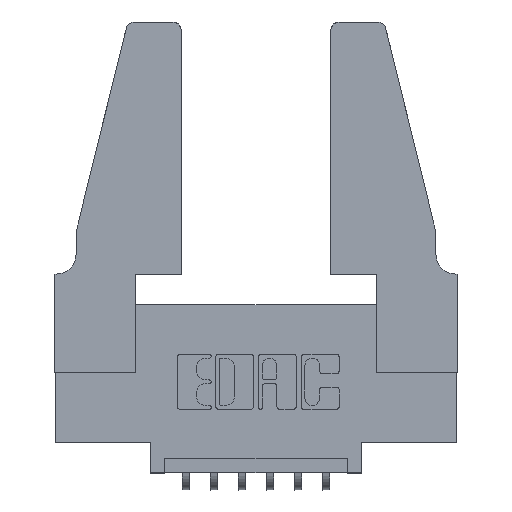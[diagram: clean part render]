
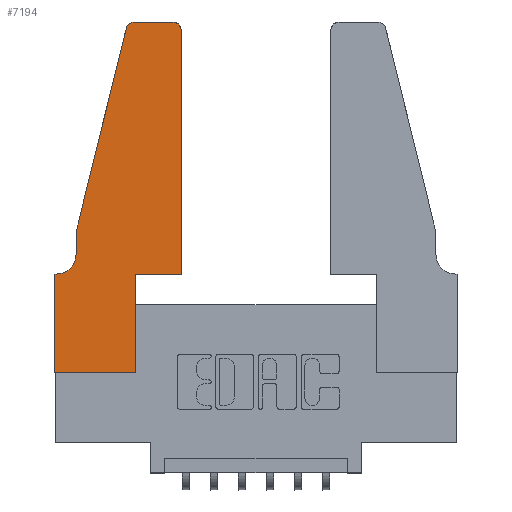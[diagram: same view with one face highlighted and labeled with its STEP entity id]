
A CAD part, top view. The second image highlights one B-rep face of the part: STEP entity #7194.
In plain terms, the highlighted planar face has unit normal (0, 0, 1).
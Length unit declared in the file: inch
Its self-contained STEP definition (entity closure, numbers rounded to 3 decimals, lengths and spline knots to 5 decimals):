
#24 = VECTOR ( 'NONE', #1150, 39.37008 ) ;
#95 = VECTOR ( 'NONE', #7363, 39.37008 ) ;
#109 = VERTEX_POINT ( 'NONE', #2676 ) ;
#180 = CARTESIAN_POINT ( 'NONE',  ( 0.25487, 1.22718, 0.37 ) ) ;
#344 = VERTEX_POINT ( 'NONE', #8142 ) ;
#568 = LINE ( 'NONE', #11033, #24 ) ;
#684 = ORIENTED_EDGE ( 'NONE', *, *, #7109, .T. ) ;
#861 = EDGE_CURVE ( 'NONE', #4608, #11034, #10524, .T. ) ;
#990 = ORIENTED_EDGE ( 'NONE', *, *, #3376, .T. ) ;
#1132 = CARTESIAN_POINT ( 'NONE',  ( 0.0755, 0.5, 0.37 ) ) ;
#1150 = DIRECTION ( 'NONE',  ( -1., 0., 0. ) ) ;
#1303 = VECTOR ( 'NONE', #10453, 39.37008 ) ;
#1322 = VERTEX_POINT ( 'NONE', #3281 ) ;
#1343 = EDGE_CURVE ( 'NONE', #11439, #109, #3256, .T. ) ;
#1404 = CARTESIAN_POINT ( 'NONE',  ( 0.4205, 1.22, 0.37 ) ) ;
#1471 = ORIENTED_EDGE ( 'NONE', *, *, #6889, .T. ) ;
#1481 = DIRECTION ( 'NONE',  ( 1., 0., 0. ) ) ;
#1549 = DIRECTION ( 'NONE',  ( 1., 0., 0. ) ) ;
#1563 = LINE ( 'NONE', #1868, #9093 ) ;
#1603 = VERTEX_POINT ( 'NONE', #1836 ) ;
#1688 = ORIENTED_EDGE ( 'NONE', *, *, #11092, .T. ) ;
#1743 = EDGE_CURVE ( 'NONE', #1603, #4608, #568, .T. ) ;
#1781 = CARTESIAN_POINT ( 'NONE',  ( 0.0755, 0.35, 0.37 ) ) ;
#1814 = EDGE_CURVE ( 'NONE', #1917, #1603, #8633, .T. ) ;
#1836 = CARTESIAN_POINT ( 'NONE',  ( 0.4205, 1.25, 0.37 ) ) ;
#1868 = CARTESIAN_POINT ( 'NONE',  ( 0., 0., 0.37 ) ) ;
#1917 = VERTEX_POINT ( 'NONE', #6999 ) ;
#2263 = CARTESIAN_POINT ( 'NONE',  ( 0.4505, 0.35, 0.37 ) ) ;
#2401 = PLANE ( 'NONE',  #6194 ) ;
#2641 = EDGE_CURVE ( 'NONE', #7543, #344, #9566, .T. ) ;
#2676 = CARTESIAN_POINT ( 'NONE',  ( 0.2865, 0., 0.37 ) ) ;
#2897 = CARTESIAN_POINT ( 'NONE',  ( 0.0755, 0.5, 0.37 ) ) ;
#2958 = VERTEX_POINT ( 'NONE', #1132 ) ;
#3074 = VERTEX_POINT ( 'NONE', #2263 ) ;
#3115 = EDGE_CURVE ( 'NONE', #109, #1322, #11562, .T. ) ;
#3256 = LINE ( 'NONE', #10674, #9085 ) ;
#3281 = CARTESIAN_POINT ( 'NONE',  ( 0.2865, 0.35, 0.37 ) ) ;
#3353 = ORIENTED_EDGE ( 'NONE', *, *, #1743, .T. ) ;
#3376 = EDGE_CURVE ( 'NONE', #2958, #7543, #3465, .T. ) ;
#3465 = LINE ( 'NONE', #2897, #95 ) ;
#3776 = EDGE_LOOP ( 'NONE', ( #3353, #9529, #4722, #990, #9411, #1471, #10688, #6001, #7278, #1688, #684, #6010 ) ) ;
#4322 = AXIS2_PLACEMENT_3D ( 'NONE', #6263, #8201, #4456 ) ;
#4456 = DIRECTION ( 'NONE',  ( -1., 0., 0. ) ) ;
#4553 = VECTOR ( 'NONE', #5973, 39.37008 ) ;
#4608 = VERTEX_POINT ( 'NONE', #6114 ) ;
#4722 = ORIENTED_EDGE ( 'NONE', *, *, #5893, .T. ) ;
#5148 = CARTESIAN_POINT ( 'NONE',  ( 0.0755, 0.5, 0.37 ) ) ;
#5365 = CARTESIAN_POINT ( 'NONE',  ( 0., 0., 0.37 ) ) ;
#5893 = EDGE_CURVE ( 'NONE', #11034, #2958, #7046, .T. ) ;
#5973 = DIRECTION ( 'NONE',  ( -0.239, -0.971, 0. ) ) ;
#6001 = ORIENTED_EDGE ( 'NONE', *, *, #1343, .T. ) ;
#6010 = ORIENTED_EDGE ( 'NONE', *, *, #1814, .T. ) ;
#6114 = CARTESIAN_POINT ( 'NONE',  ( 0.284, 1.25, 0.37 ) ) ;
#6194 = AXIS2_PLACEMENT_3D ( 'NONE', #11476, #9699, #8766 ) ;
#6263 = CARTESIAN_POINT ( 'NONE',  ( 0.0055, 0.42, 0.37 ) ) ;
#6622 = VECTOR ( 'NONE', #9454, 39.37008 ) ;
#6735 = CARTESIAN_POINT ( 'NONE',  ( 0.284, 1.22, 0.37 ) ) ;
#6889 = EDGE_CURVE ( 'NONE', #344, #8679, #9189, .T. ) ;
#6940 = DIRECTION ( 'NONE',  ( 0., 0., 1. ) ) ;
#6999 = CARTESIAN_POINT ( 'NONE',  ( 0.4505, 1.22, 0.37 ) ) ;
#7046 = LINE ( 'NONE', #5148, #4553 ) ;
#7109 = EDGE_CURVE ( 'NONE', #3074, #1917, #11454, .T. ) ;
#7194 = ADVANCED_FACE ( 'NONE', ( #7714 ), #2401, .T. ) ;
#7278 = ORIENTED_EDGE ( 'NONE', *, *, #3115, .T. ) ;
#7363 = DIRECTION ( 'NONE',  ( 0., -1., 0. ) ) ;
#7543 = VERTEX_POINT ( 'NONE', #9939 ) ;
#7698 = CARTESIAN_POINT ( 'NONE',  ( 0.4505, 0.35, 0.37 ) ) ;
#7699 = DIRECTION ( 'NONE',  ( 0., 0., 1. ) ) ;
#7714 = FACE_OUTER_BOUND ( 'NONE', #3776, .T. ) ;
#8142 = CARTESIAN_POINT ( 'NONE',  ( 0.0055, 0.35, 0.37 ) ) ;
#8201 = DIRECTION ( 'NONE',  ( 0., 0., -1. ) ) ;
#8475 = CARTESIAN_POINT ( 'NONE',  ( 0.2865, 0.35, 0.37 ) ) ;
#8633 = CIRCLE ( 'NONE', #11297, 0.03 ) ;
#8679 = VERTEX_POINT ( 'NONE', #10837 ) ;
#8766 = DIRECTION ( 'NONE',  ( 1., 0., 0. ) ) ;
#9023 = DIRECTION ( 'NONE',  ( -1., 0., 0. ) ) ;
#9085 = VECTOR ( 'NONE', #10627, 39.37008 ) ;
#9093 = VECTOR ( 'NONE', #10947, 39.37008 ) ;
#9189 = LINE ( 'NONE', #1781, #11195 ) ;
#9391 = DIRECTION ( 'NONE',  ( 0., 1., 0. ) ) ;
#9411 = ORIENTED_EDGE ( 'NONE', *, *, #2641, .T. ) ;
#9454 = DIRECTION ( 'NONE',  ( 0., 1., 0. ) ) ;
#9494 = LINE ( 'NONE', #9549, #1303 ) ;
#9529 = ORIENTED_EDGE ( 'NONE', *, *, #861, .T. ) ;
#9530 = AXIS2_PLACEMENT_3D ( 'NONE', #6735, #6940, #1549 ) ;
#9549 = CARTESIAN_POINT ( 'NONE',  ( 0.4505, 0.35, 0.37 ) ) ;
#9566 = CIRCLE ( 'NONE', #4322, 0.07 ) ;
#9699 = DIRECTION ( 'NONE',  ( 0., 0., 1. ) ) ;
#9939 = CARTESIAN_POINT ( 'NONE',  ( 0.0755, 0.42, 0.37 ) ) ;
#10453 = DIRECTION ( 'NONE',  ( 1., 0., 0. ) ) ;
#10524 = CIRCLE ( 'NONE', #9530, 0.03 ) ;
#10627 = DIRECTION ( 'NONE',  ( 1., 0., 0. ) ) ;
#10674 = CARTESIAN_POINT ( 'NONE',  ( 0., 0., 0.37 ) ) ;
#10688 = ORIENTED_EDGE ( 'NONE', *, *, #10851, .T. ) ;
#10837 = CARTESIAN_POINT ( 'NONE',  ( 0., 0.35, 0.37 ) ) ;
#10851 = EDGE_CURVE ( 'NONE', #8679, #11439, #1563, .T. ) ;
#10947 = DIRECTION ( 'NONE',  ( 0., -1., 0. ) ) ;
#11033 = CARTESIAN_POINT ( 'NONE',  ( 0.2605, 1.25, 0.37 ) ) ;
#11034 = VERTEX_POINT ( 'NONE', #180 ) ;
#11092 = EDGE_CURVE ( 'NONE', #1322, #3074, #9494, .T. ) ;
#11148 = VECTOR ( 'NONE', #9391, 39.37008 ) ;
#11195 = VECTOR ( 'NONE', #9023, 39.37008 ) ;
#11297 = AXIS2_PLACEMENT_3D ( 'NONE', #1404, #7699, #1481 ) ;
#11439 = VERTEX_POINT ( 'NONE', #5365 ) ;
#11454 = LINE ( 'NONE', #7698, #6622 ) ;
#11476 = CARTESIAN_POINT ( 'NONE',  ( 0., 0.35, 0.37 ) ) ;
#11562 = LINE ( 'NONE', #8475, #11148 ) ;
